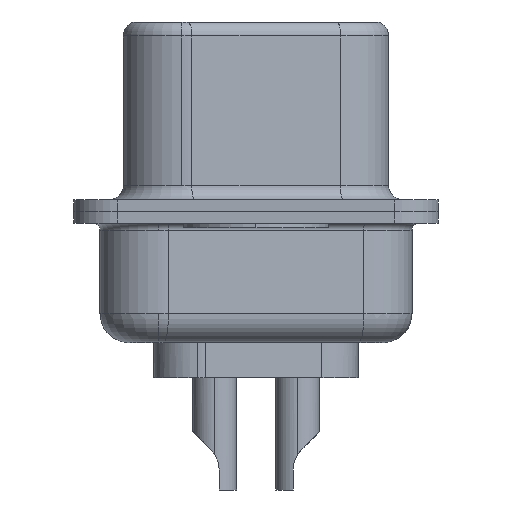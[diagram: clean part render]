
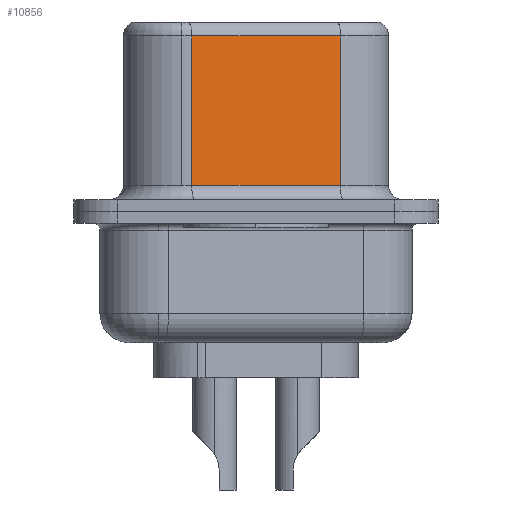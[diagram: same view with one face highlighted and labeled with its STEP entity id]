
A CAD part, left-side view. The second image highlights one B-rep face of the part: STEP entity #10856.
In plain terms, the highlighted planar face has unit normal (-0.985, -0.174, 0).
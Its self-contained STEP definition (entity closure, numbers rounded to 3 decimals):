
#9 = ORIENTED_EDGE ( 'NONE', *, *, #16088, .F. ) ;
#757 = DIRECTION ( 'NONE',  ( -0.174, 0.985, 0. ) ) ;
#894 = DIRECTION ( 'NONE',  ( 0., 0., -1. ) ) ;
#1090 = LINE ( 'NONE', #16056, #2732 ) ;
#1269 = DIRECTION ( 'NONE',  ( 0., 0., -1. ) ) ;
#2332 = CARTESIAN_POINT ( 'NONE',  ( 4.58, -2.897, 6.52 ) ) ;
#2553 = CARTESIAN_POINT ( 'NONE',  ( 4.58, -2.897, 0.9 ) ) ;
#2586 = CARTESIAN_POINT ( 'NONE',  ( 4.58, -2.897, 6.52 ) ) ;
#2732 = VECTOR ( 'NONE', #7026, 1000. ) ;
#3826 = FACE_OUTER_BOUND ( 'NONE', #13486, .T. ) ;
#3949 = CARTESIAN_POINT ( 'NONE',  ( 3.68, 2.203, 0.9 ) ) ;
#5365 = PLANE ( 'NONE',  #14793 ) ;
#6644 = CARTESIAN_POINT ( 'NONE',  ( 4.58, -2.897, 6.02 ) ) ;
#7026 = DIRECTION ( 'NONE',  ( 0.174, -0.985, 0. ) ) ;
#7864 = VECTOR ( 'NONE', #894, 1000. ) ;
#8440 = VERTEX_POINT ( 'NONE', #6644 ) ;
#8456 = LINE ( 'NONE', #9699, #17889 ) ;
#8838 = VERTEX_POINT ( 'NONE', #3949 ) ;
#9661 = DIRECTION ( 'NONE',  ( -0.174, 0.985, 0. ) ) ;
#9699 = CARTESIAN_POINT ( 'NONE',  ( 3.68, 2.203, 6.52 ) ) ;
#9717 = LINE ( 'NONE', #2332, #7864 ) ;
#9817 = CARTESIAN_POINT ( 'NONE',  ( 3.68, 2.203, 6.02 ) ) ;
#10856 = ADVANCED_FACE ( 'NONE', ( #3826 ), #5365, .F. ) ;
#11035 = VERTEX_POINT ( 'NONE', #9817 ) ;
#11744 = EDGE_CURVE ( 'NONE', #11035, #8838, #8456, .T. ) ;
#11901 = ORIENTED_EDGE ( 'NONE', *, *, #17601, .T. ) ;
#12572 = DIRECTION ( 'NONE',  ( 0.985, 0.174, 0. ) ) ;
#12720 = VECTOR ( 'NONE', #9661, 1000. ) ;
#12746 = CARTESIAN_POINT ( 'NONE',  ( 4.58, -2.897, 6.02 ) ) ;
#12911 = ORIENTED_EDGE ( 'NONE', *, *, #11744, .T. ) ;
#13157 = ORIENTED_EDGE ( 'NONE', *, *, #14021, .T. ) ;
#13486 = EDGE_LOOP ( 'NONE', ( #9, #13157, #12911, #11901 ) ) ;
#14021 = EDGE_CURVE ( 'NONE', #8440, #11035, #14093, .T. ) ;
#14093 = LINE ( 'NONE', #12746, #12720 ) ;
#14793 = AXIS2_PLACEMENT_3D ( 'NONE', #2586, #12572, #757 ) ;
#16056 = CARTESIAN_POINT ( 'NONE',  ( 4.58, -2.897, 0.9 ) ) ;
#16088 = EDGE_CURVE ( 'NONE', #8440, #16934, #9717, .T. ) ;
#16934 = VERTEX_POINT ( 'NONE', #2553 ) ;
#17601 = EDGE_CURVE ( 'NONE', #8838, #16934, #1090, .T. ) ;
#17889 = VECTOR ( 'NONE', #1269, 1000. ) ;
